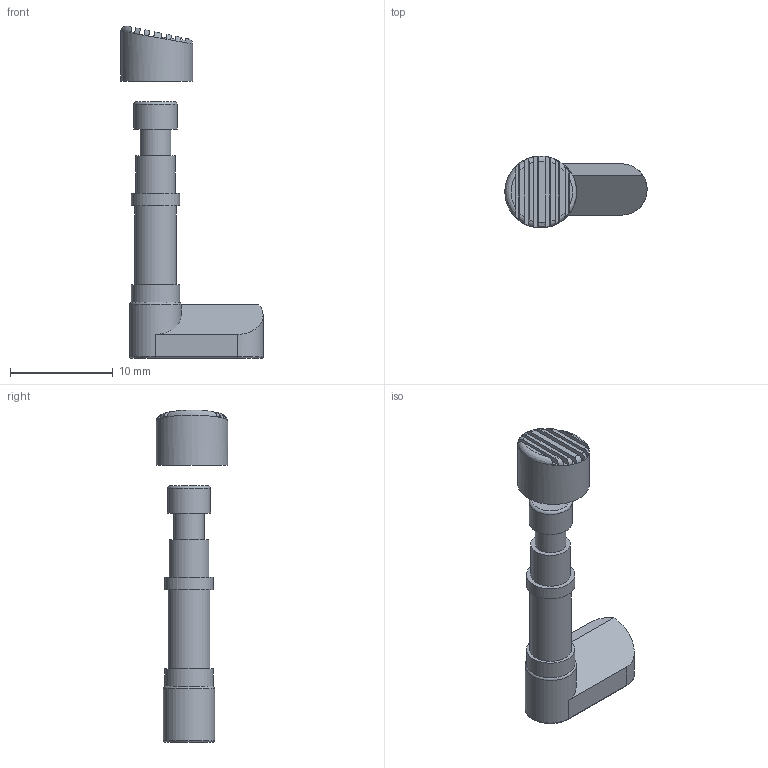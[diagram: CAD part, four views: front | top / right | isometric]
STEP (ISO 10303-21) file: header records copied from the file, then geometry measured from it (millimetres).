
FILE_DESCRIPTION(/* description */ (''),/* implementation_level */ '2;1');
FILE_NAME(/* name */ 'C9-mag-release v7.step',/* time_stamp */ '2021-03-10T06:17:40-08:00',/* author */ (''),/* organization */ (''),/* preprocessor_version */ 'ST-DEVELOPER v18.1',/* originating_system */ 'Autodesk Translation Framework v9.7.1.1290',/* authorisation */ '');
FILE_SCHEMA (('AUTOMOTIVE_DESIGN { 1 0 10303 214 3 1 1 }'));
Length unit declared in the file: millimetre
Products named in the file (1): C9-mag-release
Bounding box: 13.88 x 7 x 32.37 mm (x, y, z)
Volume: 644.1 mm3; surface area: 902.3 mm2
Topology: 3 solids, 3 shells, 239 faces, 655 edges, 429 vertices
Faces by surface type: plane 199, cylinder 29, torus 8, bspline 2, cone 1
Full cylindrical faces by diameter (mm): 2.7 x1, 3 x1, 3.87 x1, 4.08 x1, 4.2 x2, 4.7 x1, 4.74 x1, 5 x1, 7 x1
Entity records: 8529 total; most frequent: CARTESIAN_POINT 2418, ORIENTED_EDGE 1310, DIRECTION 1217, EDGE_CURVE 655, LINE 453, VECTOR 453, VERTEX_POINT 429, AXIS2_PLACEMENT_3D 382
